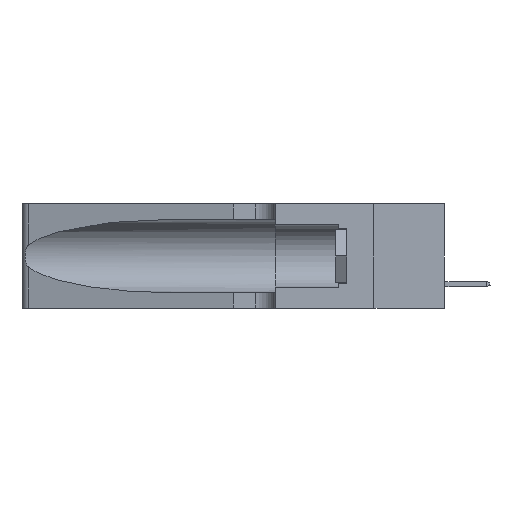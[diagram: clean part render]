
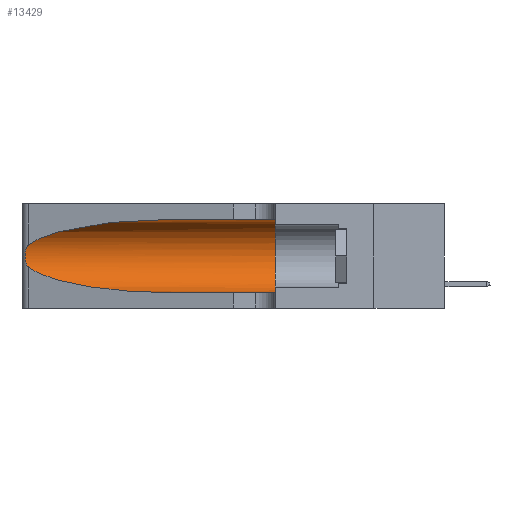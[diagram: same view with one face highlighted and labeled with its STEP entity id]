
A CAD part, left-side view. The second image highlights one B-rep face of the part: STEP entity #13429.
In plain terms, the highlighted cylindrical face has radius 3.308 mm (diameter 6.617 mm), a partial arc.
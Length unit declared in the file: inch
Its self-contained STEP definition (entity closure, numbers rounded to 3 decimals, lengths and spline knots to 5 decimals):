
#140 = CARTESIAN_POINT ( 'NONE',  ( 0.25487, 1.22718, 0.22369 ) ) ;
#420 = VERTEX_POINT ( 'NONE', #12090 ) ;
#495 = CARTESIAN_POINT ( 'NONE',  ( 0.25487, 1.22718, 0.14631 ) ) ;
#1045 = AXIS2_PLACEMENT_3D ( 'NONE', #9903, #12611, #11212 ) ;
#1082 = EDGE_CURVE ( 'NONE', #1205, #10775, #17602, .T. ) ;
#1205 = VERTEX_POINT ( 'NONE', #4584 ) ;
#1790 = DIRECTION ( 'NONE',  ( 0., -1., 0. ) ) ;
#1917 = DIRECTION ( 'NONE',  ( 0., 0., -1. ) ) ;
#1920 = VECTOR ( 'NONE', #1790, 39.37008 ) ;
#1973 = CARTESIAN_POINT ( 'NONE',  ( 0.25487, 1.22718, 0.22369 ) ) ;
#2030 = CARTESIAN_POINT ( 'NONE',  ( 0.1305, 0.35, 0.31525 ) ) ;
#2516 =( BOUNDED_CURVE ( )  B_SPLINE_CURVE ( 3, ( #5626, #6989, #16593, #140 ),
 .UNSPECIFIED., .F., .T. ) 
 B_SPLINE_CURVE_WITH_KNOTS ( ( 4, 4 ),
 ( 1.5708, 2.84003 ),
 .UNSPECIFIED. ) 
 CURVE ( )  GEOMETRIC_REPRESENTATION_ITEM ( )  RATIONAL_B_SPLINE_CURVE ( ( 1., 0.87, 0.87, 1. ) ) 
 REPRESENTATION_ITEM ( '' )  );
#2871 = EDGE_CURVE ( 'NONE', #1205, #8647, #2516, .T. ) ;
#3415 = CARTESIAN_POINT ( 'NONE',  ( 0.1305, 1.61858, 0.185 ) ) ;
#3546 = FACE_OUTER_BOUND ( 'NONE', #15495, .T. ) ;
#3697 = ORIENTED_EDGE ( 'NONE', *, *, #5856, .T. ) ;
#4277 = ORIENTED_EDGE ( 'NONE', *, *, #1082, .F. ) ;
#4504 = CARTESIAN_POINT ( 'NONE',  ( 0.18966, 0.96281, 0.05475 ) ) ;
#4584 = CARTESIAN_POINT ( 'NONE',  ( 0.1305, 0.72297, 0.31525 ) ) ;
#4828 = CARTESIAN_POINT ( 'NONE',  ( 0.26075, 1.23896, 0.19203 ) ) ;
#4997 = CIRCLE ( 'NONE', #1045, 0.13025 ) ;
#5082 = EDGE_CURVE ( 'NONE', #420, #14593, #7938, .T. ) ;
#5626 = CARTESIAN_POINT ( 'NONE',  ( 0.1305, 0.72297, 0.31525 ) ) ;
#5722 = CARTESIAN_POINT ( 'NONE',  ( 0.25854, 1.2359, 0.20912 ) ) ;
#5766 = CARTESIAN_POINT ( 'NONE',  ( 0.1305, 0.35, 0.05475 ) ) ;
#5856 = EDGE_CURVE ( 'NONE', #8647, #10176, #13203, .T. ) ;
#6097 = CARTESIAN_POINT ( 'NONE',  ( 0.25639, 1.23186, 0.15144 ) ) ;
#6463 = EDGE_CURVE ( 'NONE', #10176, #420, #6581, .T. ) ;
#6581 =( BOUNDED_CURVE ( )  B_SPLINE_CURVE ( 3, ( #495, #7372, #4504, #17045 ),
 .UNSPECIFIED., .F., .F. ) 
 B_SPLINE_CURVE_WITH_KNOTS ( ( 4, 4 ),
 ( 3.44316, 4.71239 ),
 .UNSPECIFIED. ) 
 CURVE ( )  GEOMETRIC_REPRESENTATION_ITEM ( )  RATIONAL_B_SPLINE_CURVE ( ( 1., 0.87, 0.87, 1. ) ) 
 REPRESENTATION_ITEM ( '' )  );
#6674 = CARTESIAN_POINT ( 'NONE',  ( 0.25856, 1.23593, 0.16098 ) ) ;
#6777 = AXIS2_PLACEMENT_3D ( 'NONE', #3415, #12859, #1917 ) ;
#6989 = CARTESIAN_POINT ( 'NONE',  ( 0.18966, 0.96281, 0.31525 ) ) ;
#7051 = DIRECTION ( 'NONE',  ( 0., -1., 0. ) ) ;
#7372 = CARTESIAN_POINT ( 'NONE',  ( 0.2373, 1.15595, 0.08982 ) ) ;
#7938 = LINE ( 'NONE', #11457, #1920 ) ;
#8647 = VERTEX_POINT ( 'NONE', #9619 ) ;
#9339 = CARTESIAN_POINT ( 'NONE',  ( 0.26017, 1.23833, 0.17102 ) ) ;
#9433 = EDGE_CURVE ( 'NONE', #10775, #14593, #4997, .T. ) ;
#9619 = CARTESIAN_POINT ( 'NONE',  ( 0.25487, 1.22718, 0.22369 ) ) ;
#9903 = CARTESIAN_POINT ( 'NONE',  ( 0.1305, 0.35, 0.185 ) ) ;
#10176 = VERTEX_POINT ( 'NONE', #15349 ) ;
#10335 = CARTESIAN_POINT ( 'NONE',  ( 0.25639, 1.23184, 0.21858 ) ) ;
#10775 = VERTEX_POINT ( 'NONE', #2030 ) ;
#11212 = DIRECTION ( 'NONE',  ( 0., 0., 1. ) ) ;
#11251 = CARTESIAN_POINT ( 'NONE',  ( 0.25789, 1.23486, 0.15765 ) ) ;
#11457 = CARTESIAN_POINT ( 'NONE',  ( 0.1305, 1.61858, 0.05475 ) ) ;
#11673 = CARTESIAN_POINT ( 'NONE',  ( 0.25555, 1.22993, 0.14849 ) ) ;
#11929 = CYLINDRICAL_SURFACE ( 'NONE', #6777, 0.13025 ) ;
#12090 = CARTESIAN_POINT ( 'NONE',  ( 0.1305, 0.72297, 0.05475 ) ) ;
#12230 = ORIENTED_EDGE ( 'NONE', *, *, #5082, .T. ) ;
#12611 = DIRECTION ( 'NONE',  ( 0., 1., 0. ) ) ;
#12685 = ORIENTED_EDGE ( 'NONE', *, *, #2871, .T. ) ;
#12859 = DIRECTION ( 'NONE',  ( 0., -1., 0. ) ) ;
#13057 = CARTESIAN_POINT ( 'NONE',  ( 0.26018, 1.23835, 0.19895 ) ) ;
#13177 = ORIENTED_EDGE ( 'NONE', *, *, #9433, .F. ) ;
#13203 = B_SPLINE_CURVE_WITH_KNOTS ( 'NONE', 3,
 ( #1973, #15773, #10335, #13743, #5722, #13057, #4828, #15799, #9339, #6674, #11251, #6097, #11673, #15721 ),
 .UNSPECIFIED., .F., .F.,
 ( 4, 2, 2, 2, 2, 2, 4 ),
 ( 0., 0.00027, 0.00053, 0.00107, 0.0016, 0.00187, 0.00214 ),
 .UNSPECIFIED. ) ;
#13429 = ADVANCED_FACE ( 'NONE', ( #3546 ), #11929, .F. ) ;
#13743 = CARTESIAN_POINT ( 'NONE',  ( 0.25787, 1.23484, 0.2124 ) ) ;
#13978 = VECTOR ( 'NONE', #7051, 39.37008 ) ;
#14593 = VERTEX_POINT ( 'NONE', #5766 ) ;
#15283 = CARTESIAN_POINT ( 'NONE',  ( 0.1305, 1.61858, 0.31525 ) ) ;
#15349 = CARTESIAN_POINT ( 'NONE',  ( 0.25487, 1.22718, 0.14631 ) ) ;
#15495 = EDGE_LOOP ( 'NONE', ( #12685, #3697, #15643, #12230, #13177, #4277 ) ) ;
#15643 = ORIENTED_EDGE ( 'NONE', *, *, #6463, .T. ) ;
#15721 = CARTESIAN_POINT ( 'NONE',  ( 0.25487, 1.22718, 0.14631 ) ) ;
#15773 = CARTESIAN_POINT ( 'NONE',  ( 0.25555, 1.22994, 0.2215 ) ) ;
#15799 = CARTESIAN_POINT ( 'NONE',  ( 0.26075, 1.23896, 0.178 ) ) ;
#16593 = CARTESIAN_POINT ( 'NONE',  ( 0.2373, 1.15595, 0.28018 ) ) ;
#17045 = CARTESIAN_POINT ( 'NONE',  ( 0.1305, 0.72297, 0.05475 ) ) ;
#17602 = LINE ( 'NONE', #15283, #13978 ) ;
